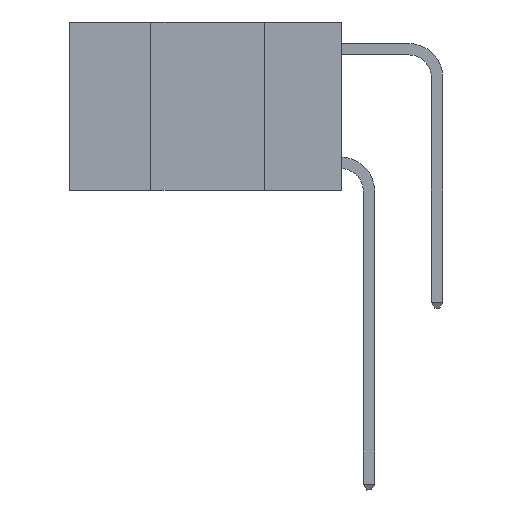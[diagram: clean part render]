
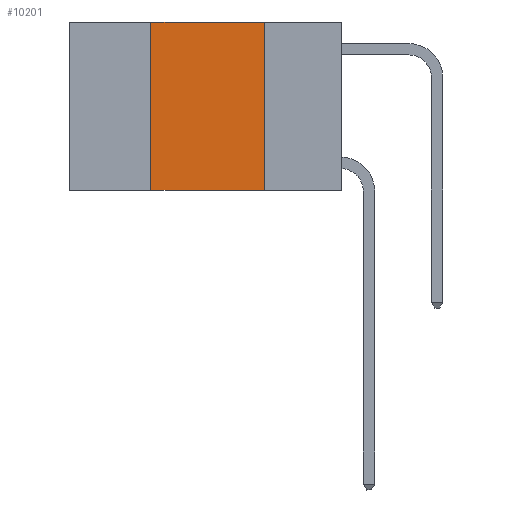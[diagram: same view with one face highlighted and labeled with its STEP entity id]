
A CAD part, left-side view. The second image highlights one B-rep face of the part: STEP entity #10201.
In plain terms, the highlighted planar face has unit normal (-1, 0, 0).
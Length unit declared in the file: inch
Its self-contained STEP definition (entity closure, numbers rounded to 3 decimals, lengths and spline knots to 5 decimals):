
#97 = VERTEX_POINT ( 'NONE', #3656 ) ;
#1873 = VERTEX_POINT ( 'NONE', #14131 ) ;
#2080 = VECTOR ( 'NONE', #4103, 39.37008 ) ;
#2222 = DIRECTION ( 'NONE',  ( 0., 0., -1. ) ) ;
#2733 = EDGE_CURVE ( 'NONE', #1873, #8901, #7568, .T. ) ;
#3569 = EDGE_CURVE ( 'NONE', #97, #6942, #5788, .T. ) ;
#3656 = CARTESIAN_POINT ( 'NONE',  ( 0., 0.42, -0.37 ) ) ;
#4103 = DIRECTION ( 'NONE',  ( 0., -1., 0. ) ) ;
#4152 = EDGE_LOOP ( 'NONE', ( #13681, #14060, #11220, #8399 ) ) ;
#4788 = CARTESIAN_POINT ( 'NONE',  ( 0., 0.6, 0. ) ) ;
#5788 = LINE ( 'NONE', #12597, #6179 ) ;
#6043 = DIRECTION ( 'NONE',  ( 0., 0., -1. ) ) ;
#6179 = VECTOR ( 'NONE', #10181, 39.37008 ) ;
#6484 = CARTESIAN_POINT ( 'NONE',  ( 0., 0.17, -0.37 ) ) ;
#6766 = FACE_OUTER_BOUND ( 'NONE', #4152, .T. ) ;
#6831 = LINE ( 'NONE', #10212, #12953 ) ;
#6942 = VERTEX_POINT ( 'NONE', #11522 ) ;
#7568 = LINE ( 'NONE', #8523, #13659 ) ;
#8399 = ORIENTED_EDGE ( 'NONE', *, *, #13753, .T. ) ;
#8523 = CARTESIAN_POINT ( 'NONE',  ( 0., 0.17, 0. ) ) ;
#8739 = LINE ( 'NONE', #15124, #2080 ) ;
#8901 = VERTEX_POINT ( 'NONE', #6484 ) ;
#10181 = DIRECTION ( 'NONE',  ( 0., 0., 1. ) ) ;
#10201 = ADVANCED_FACE ( 'NONE', ( #6766 ), #12147, .F. ) ;
#10212 = CARTESIAN_POINT ( 'NONE',  ( 0., 0.6, 0. ) ) ;
#11220 = ORIENTED_EDGE ( 'NONE', *, *, #3569, .F. ) ;
#11522 = CARTESIAN_POINT ( 'NONE',  ( 0., 0.42, 0. ) ) ;
#11674 = EDGE_CURVE ( 'NONE', #6942, #1873, #6831, .T. ) ;
#12147 = PLANE ( 'NONE',  #14153 ) ;
#12597 = CARTESIAN_POINT ( 'NONE',  ( 0., 0.42, 0. ) ) ;
#12953 = VECTOR ( 'NONE', #13838, 39.37008 ) ;
#13372 = DIRECTION ( 'NONE',  ( 1., 0., 0. ) ) ;
#13659 = VECTOR ( 'NONE', #2222, 39.37008 ) ;
#13681 = ORIENTED_EDGE ( 'NONE', *, *, #2733, .F. ) ;
#13753 = EDGE_CURVE ( 'NONE', #97, #8901, #8739, .T. ) ;
#13838 = DIRECTION ( 'NONE',  ( 0., -1., 0. ) ) ;
#14060 = ORIENTED_EDGE ( 'NONE', *, *, #11674, .F. ) ;
#14131 = CARTESIAN_POINT ( 'NONE',  ( 0., 0.17, 0. ) ) ;
#14153 = AXIS2_PLACEMENT_3D ( 'NONE', #4788, #13372, #6043 ) ;
#15124 = CARTESIAN_POINT ( 'NONE',  ( 0., 0.6, -0.37 ) ) ;
